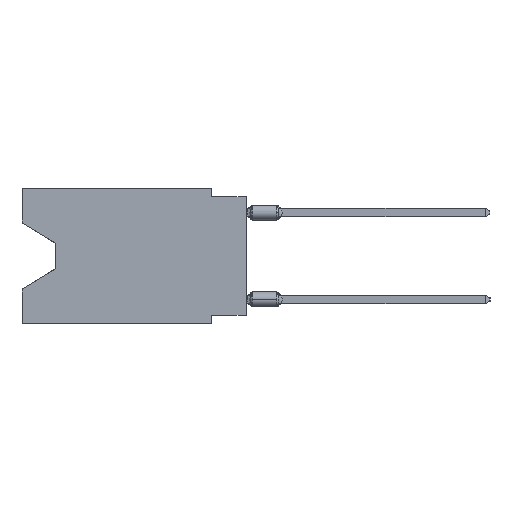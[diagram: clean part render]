
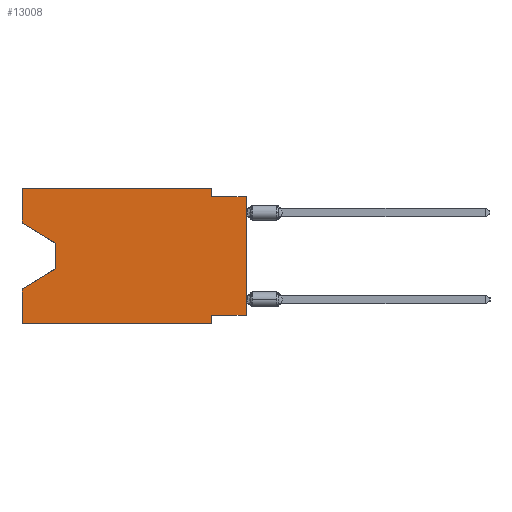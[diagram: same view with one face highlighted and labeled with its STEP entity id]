
A CAD part, left-side view. The second image highlights one B-rep face of the part: STEP entity #13008.
In plain terms, the highlighted planar face has unit normal (-1, 0, 0).
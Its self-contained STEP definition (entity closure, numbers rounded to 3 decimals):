
#53 = ORIENTED_EDGE ( 'NONE', *, *, #12496, .T. ) ;
#961 = VECTOR ( 'NONE', #43249, 1000. ) ;
#1042 = EDGE_CURVE ( 'NONE', #35593, #16758, #2748, .T. ) ;
#1217 = VECTOR ( 'NONE', #45041, 1000. ) ;
#1318 = VECTOR ( 'NONE', #9093, 1000. ) ;
#1539 = CARTESIAN_POINT ( 'NONE',  ( 0., 16.383, 0. ) ) ;
#1869 = LINE ( 'NONE', #18796, #961 ) ;
#2089 = LINE ( 'NONE', #26339, #3116 ) ;
#2188 = LINE ( 'NONE', #12485, #43943 ) ;
#2274 = VERTEX_POINT ( 'NONE', #2523 ) ;
#2523 = CARTESIAN_POINT ( 'NONE',  ( 0., 16.383, -7.36 ) ) ;
#2748 = LINE ( 'NONE', #13933, #25151 ) ;
#2863 = ORIENTED_EDGE ( 'NONE', *, *, #1042, .F. ) ;
#3116 = VECTOR ( 'NONE', #23137, 1000. ) ;
#3444 = VERTEX_POINT ( 'NONE', #25488 ) ;
#5081 = CARTESIAN_POINT ( 'NONE',  ( 0., 16.383, 0. ) ) ;
#5203 = VERTEX_POINT ( 'NONE', #15503 ) ;
#8386 = CARTESIAN_POINT ( 'NONE',  ( 0., 2.54, -9.271 ) ) ;
#9081 = FACE_OUTER_BOUND ( 'NONE', #15715, .T. ) ;
#9093 = DIRECTION ( 'NONE',  ( 0., 0., -1. ) ) ;
#9850 = CARTESIAN_POINT ( 'NONE',  ( 0., 2.54, -9.906 ) ) ;
#10257 = CARTESIAN_POINT ( 'NONE',  ( 0., 0., -0.635 ) ) ;
#10436 = CARTESIAN_POINT ( 'NONE',  ( 0., 16.383, -9.906 ) ) ;
#10487 = LINE ( 'NONE', #44810, #1217 ) ;
#11124 = CARTESIAN_POINT ( 'NONE',  ( 0., 0., -9.271 ) ) ;
#11364 = DIRECTION ( 'NONE',  ( 0., 1., 0. ) ) ;
#11426 = VERTEX_POINT ( 'NONE', #20545 ) ;
#11618 = VERTEX_POINT ( 'NONE', #8386 ) ;
#11979 = ORIENTED_EDGE ( 'NONE', *, *, #29552, .F. ) ;
#12295 = PLANE ( 'NONE',  #25061 ) ;
#12485 = CARTESIAN_POINT ( 'NONE',  ( 0., 16.383, 0. ) ) ;
#12496 = EDGE_CURVE ( 'NONE', #35593, #40968, #2089, .T. ) ;
#12575 = EDGE_CURVE ( 'NONE', #5203, #11426, #1869, .T. ) ;
#12648 = EDGE_CURVE ( 'NONE', #11618, #18727, #23355, .T. ) ;
#12863 = LINE ( 'NONE', #26824, #14406 ) ;
#12966 = DIRECTION ( 'NONE',  ( 1., 0., 0. ) ) ;
#13008 = ADVANCED_FACE ( 'NONE', ( #9081 ), #12295, .F. ) ;
#13088 = VECTOR ( 'NONE', #11364, 1000. ) ;
#13116 = VERTEX_POINT ( 'NONE', #10436 ) ;
#13933 = CARTESIAN_POINT ( 'NONE',  ( 0., 16.383, 0. ) ) ;
#14406 = VECTOR ( 'NONE', #40754, 1000. ) ;
#15503 = CARTESIAN_POINT ( 'NONE',  ( 0., 2.54, 0. ) ) ;
#15565 = CARTESIAN_POINT ( 'NONE',  ( 0., 13.97, -4.013 ) ) ;
#15715 = EDGE_LOOP ( 'NONE', ( #53, #32497, #43735, #30946, #20412, #27998, #11979, #35493, #31833, #42511, #21251, #2863 ) ) ;
#16673 = CARTESIAN_POINT ( 'NONE',  ( 0., 16.383, -2.546 ) ) ;
#16758 = VERTEX_POINT ( 'NONE', #5081 ) ;
#18727 = VERTEX_POINT ( 'NONE', #24003 ) ;
#18796 = CARTESIAN_POINT ( 'NONE',  ( 0., 2.54, 0. ) ) ;
#20074 = CARTESIAN_POINT ( 'NONE',  ( 0., 13.97, -4.013 ) ) ;
#20134 = DIRECTION ( 'NONE',  ( 0., 0., 1. ) ) ;
#20243 = EDGE_CURVE ( 'NONE', #40968, #3444, #40422, .T. ) ;
#20412 = ORIENTED_EDGE ( 'NONE', *, *, #25728, .T. ) ;
#20545 = CARTESIAN_POINT ( 'NONE',  ( 0., 2.54, -0.635 ) ) ;
#21251 = ORIENTED_EDGE ( 'NONE', *, *, #43105, .F. ) ;
#21402 = VECTOR ( 'NONE', #34093, 1000. ) ;
#23137 = DIRECTION ( 'NONE',  ( 0., -0.855, -0.519 ) ) ;
#23355 = LINE ( 'NONE', #9850, #21402 ) ;
#24003 = CARTESIAN_POINT ( 'NONE',  ( 0., 2.54, -9.906 ) ) ;
#25061 = AXIS2_PLACEMENT_3D ( 'NONE', #1539, #12966, #33104 ) ;
#25151 = VECTOR ( 'NONE', #20134, 1000. ) ;
#25488 = CARTESIAN_POINT ( 'NONE',  ( 0., 13.97, -5.893 ) ) ;
#25728 = EDGE_CURVE ( 'NONE', #13116, #18727, #35328, .T. ) ;
#26339 = CARTESIAN_POINT ( 'NONE',  ( 0., 16.383, -2.546 ) ) ;
#26392 = CARTESIAN_POINT ( 'NONE',  ( 0., 0., -0.635 ) ) ;
#26824 = CARTESIAN_POINT ( 'NONE',  ( 0., 13.97, -5.893 ) ) ;
#26830 = DIRECTION ( 'NONE',  ( 0., 0., 1. ) ) ;
#27052 = LINE ( 'NONE', #34350, #36428 ) ;
#27995 = VECTOR ( 'NONE', #41367, 1000. ) ;
#27998 = ORIENTED_EDGE ( 'NONE', *, *, #12648, .F. ) ;
#29119 = EDGE_CURVE ( 'NONE', #13116, #2274, #27052, .T. ) ;
#29552 = EDGE_CURVE ( 'NONE', #33684, #11618, #42681, .T. ) ;
#30089 = DIRECTION ( 'NONE',  ( 0., -1., 0. ) ) ;
#30946 = ORIENTED_EDGE ( 'NONE', *, *, #29119, .F. ) ;
#31239 = CARTESIAN_POINT ( 'NONE',  ( 0., 16.383, -9.906 ) ) ;
#31470 = VERTEX_POINT ( 'NONE', #26392 ) ;
#31833 = ORIENTED_EDGE ( 'NONE', *, *, #35837, .F. ) ;
#32497 = ORIENTED_EDGE ( 'NONE', *, *, #20243, .T. ) ;
#33104 = DIRECTION ( 'NONE',  ( 0., 0., -1. ) ) ;
#33684 = VERTEX_POINT ( 'NONE', #34610 ) ;
#34093 = DIRECTION ( 'NONE',  ( 0., 0., -1. ) ) ;
#34350 = CARTESIAN_POINT ( 'NONE',  ( 0., 16.383, 0. ) ) ;
#34610 = CARTESIAN_POINT ( 'NONE',  ( 0., 0., -9.271 ) ) ;
#35328 = LINE ( 'NONE', #31239, #37938 ) ;
#35493 = ORIENTED_EDGE ( 'NONE', *, *, #40011, .T. ) ;
#35593 = VERTEX_POINT ( 'NONE', #16673 ) ;
#35837 = EDGE_CURVE ( 'NONE', #11426, #31470, #41586, .T. ) ;
#36428 = VECTOR ( 'NONE', #26830, 1000. ) ;
#37938 = VECTOR ( 'NONE', #45196, 1000. ) ;
#40011 = EDGE_CURVE ( 'NONE', #33684, #31470, #10487, .T. ) ;
#40422 = LINE ( 'NONE', #20074, #1318 ) ;
#40637 = EDGE_CURVE ( 'NONE', #3444, #2274, #12863, .T. ) ;
#40754 = DIRECTION ( 'NONE',  ( 0., 0.855, -0.519 ) ) ;
#40968 = VERTEX_POINT ( 'NONE', #15565 ) ;
#41367 = DIRECTION ( 'NONE',  ( 0., -1., 0. ) ) ;
#41586 = LINE ( 'NONE', #10257, #27995 ) ;
#42511 = ORIENTED_EDGE ( 'NONE', *, *, #12575, .F. ) ;
#42681 = LINE ( 'NONE', #11124, #13088 ) ;
#43105 = EDGE_CURVE ( 'NONE', #16758, #5203, #2188, .T. ) ;
#43249 = DIRECTION ( 'NONE',  ( 0., 0., -1. ) ) ;
#43735 = ORIENTED_EDGE ( 'NONE', *, *, #40637, .T. ) ;
#43943 = VECTOR ( 'NONE', #30089, 1000. ) ;
#44810 = CARTESIAN_POINT ( 'NONE',  ( 0., 0., 0. ) ) ;
#45041 = DIRECTION ( 'NONE',  ( 0., 0., 1. ) ) ;
#45196 = DIRECTION ( 'NONE',  ( 0., -1., 0. ) ) ;
